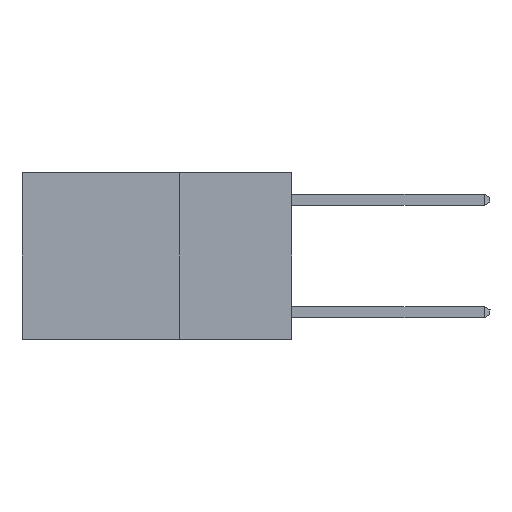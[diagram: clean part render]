
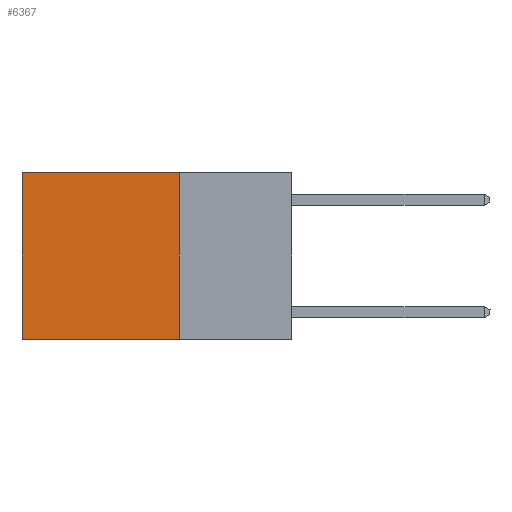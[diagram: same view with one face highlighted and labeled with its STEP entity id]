
A CAD part, left-side view. The second image highlights one B-rep face of the part: STEP entity #6367.
In plain terms, the highlighted planar face has unit normal (-1, 0, 0).
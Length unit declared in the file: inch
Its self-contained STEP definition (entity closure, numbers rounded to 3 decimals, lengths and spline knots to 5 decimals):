
#71 = EDGE_CURVE ( 'NONE', #1378, #8306, #4929, .T. ) ;
#534 = CARTESIAN_POINT ( 'NONE',  ( 0.2625, 0.6, 0. ) ) ;
#1274 = LINE ( 'NONE', #534, #4925 ) ;
#1365 = CARTESIAN_POINT ( 'NONE',  ( 0.2625, 0.25, 0. ) ) ;
#1378 = VERTEX_POINT ( 'NONE', #9707 ) ;
#1384 = DIRECTION ( 'NONE',  ( 0., 0., -1. ) ) ;
#2151 = VECTOR ( 'NONE', #1384, 39.37008 ) ;
#2323 = VECTOR ( 'NONE', #3572, 39.37008 ) ;
#2676 = CARTESIAN_POINT ( 'NONE',  ( 0.2625, 0.25, 0. ) ) ;
#2710 = EDGE_LOOP ( 'NONE', ( #5134, #7658, #7663, #5158 ) ) ;
#2980 = DIRECTION ( 'NONE',  ( 1., 0., 0. ) ) ;
#3013 = DIRECTION ( 'NONE',  ( 0., 0., -1. ) ) ;
#3051 = VECTOR ( 'NONE', #4642, 39.37008 ) ;
#3448 = LINE ( 'NONE', #6245, #3051 ) ;
#3572 = DIRECTION ( 'NONE',  ( 0., 1., 0. ) ) ;
#3792 = PLANE ( 'NONE',  #9628 ) ;
#4642 = DIRECTION ( 'NONE',  ( 0., 1., 0. ) ) ;
#4723 = VERTEX_POINT ( 'NONE', #10163 ) ;
#4925 = VECTOR ( 'NONE', #7950, 39.37008 ) ;
#4929 = LINE ( 'NONE', #2676, #2151 ) ;
#4932 = EDGE_CURVE ( 'NONE', #10450, #4723, #1274, .T. ) ;
#5134 = ORIENTED_EDGE ( 'NONE', *, *, #4932, .T. ) ;
#5158 = ORIENTED_EDGE ( 'NONE', *, *, #10235, .T. ) ;
#5964 = CARTESIAN_POINT ( 'NONE',  ( 0.2625, 0.25, -0.37 ) ) ;
#6245 = CARTESIAN_POINT ( 'NONE',  ( 0.2625, 0.25, 0. ) ) ;
#6367 = ADVANCED_FACE ( 'NONE', ( #6405 ), #3792, .F. ) ;
#6405 = FACE_OUTER_BOUND ( 'NONE', #2710, .T. ) ;
#7105 = CARTESIAN_POINT ( 'NONE',  ( 0.2625, 0.25, -0.37 ) ) ;
#7658 = ORIENTED_EDGE ( 'NONE', *, *, #8214, .F. ) ;
#7663 = ORIENTED_EDGE ( 'NONE', *, *, #71, .F. ) ;
#7950 = DIRECTION ( 'NONE',  ( 0., 0., -1. ) ) ;
#8214 = EDGE_CURVE ( 'NONE', #8306, #4723, #10426, .T. ) ;
#8306 = VERTEX_POINT ( 'NONE', #7105 ) ;
#8547 = CARTESIAN_POINT ( 'NONE',  ( 0.2625, 0.6, 0. ) ) ;
#9628 = AXIS2_PLACEMENT_3D ( 'NONE', #1365, #2980, #3013 ) ;
#9707 = CARTESIAN_POINT ( 'NONE',  ( 0.2625, 0.25, 0. ) ) ;
#10163 = CARTESIAN_POINT ( 'NONE',  ( 0.2625, 0.6, -0.37 ) ) ;
#10235 = EDGE_CURVE ( 'NONE', #1378, #10450, #3448, .T. ) ;
#10426 = LINE ( 'NONE', #5964, #2323 ) ;
#10450 = VERTEX_POINT ( 'NONE', #8547 ) ;
